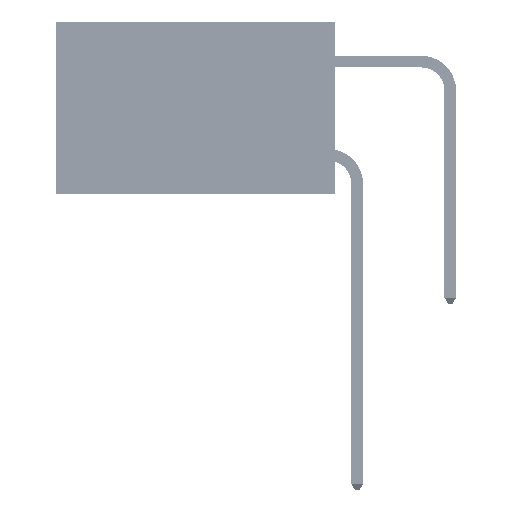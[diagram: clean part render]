
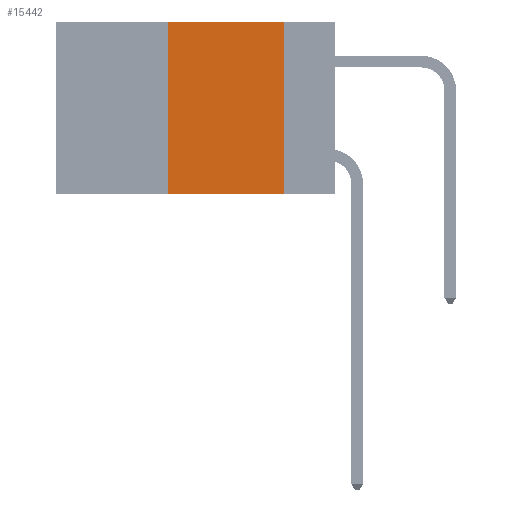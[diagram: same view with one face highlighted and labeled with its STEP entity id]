
A CAD part, left-side view. The second image highlights one B-rep face of the part: STEP entity #15442.
In plain terms, the highlighted planar face has unit normal (-1, 0, 0).
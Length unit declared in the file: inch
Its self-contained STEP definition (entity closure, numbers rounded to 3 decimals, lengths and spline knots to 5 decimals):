
#2780 = DIRECTION ( 'NONE',  ( 0., 0., 1. ) ) ;
#3039 = CARTESIAN_POINT ( 'NONE',  ( 0., 0.6, -0.37 ) ) ;
#4816 = CARTESIAN_POINT ( 'NONE',  ( 0., 0.36, -0.37 ) ) ;
#5075 = CARTESIAN_POINT ( 'NONE',  ( 0., 0.6, 0. ) ) ;
#6278 = VECTOR ( 'NONE', #37087, 39.37008 ) ;
#7468 = CARTESIAN_POINT ( 'NONE',  ( 0., 0.36, 0. ) ) ;
#8004 = CARTESIAN_POINT ( 'NONE',  ( 0., 0.11, -0.37 ) ) ;
#8449 = EDGE_LOOP ( 'NONE', ( #29935, #36729, #36062, #20959 ) ) ;
#8723 = DIRECTION ( 'NONE',  ( 1., 0., 0. ) ) ;
#8967 = FACE_OUTER_BOUND ( 'NONE', #8449, .T. ) ;
#9272 = VECTOR ( 'NONE', #2780, 39.37008 ) ;
#11995 = EDGE_CURVE ( 'NONE', #47889, #17539, #29775, .T. ) ;
#12597 = AXIS2_PLACEMENT_3D ( 'NONE', #16553, #8723, #31439 ) ;
#14739 = VECTOR ( 'NONE', #44502, 39.37008 ) ;
#15414 = EDGE_CURVE ( 'NONE', #46195, #47889, #27761, .T. ) ;
#15442 = ADVANCED_FACE ( 'NONE', ( #8967 ), #35083, .F. ) ;
#16553 = CARTESIAN_POINT ( 'NONE',  ( 0., 0.6, 0. ) ) ;
#17539 = VERTEX_POINT ( 'NONE', #8004 ) ;
#20959 = ORIENTED_EDGE ( 'NONE', *, *, #37553, .T. ) ;
#21568 = LINE ( 'NONE', #36219, #9272 ) ;
#25056 = VECTOR ( 'NONE', #39238, 39.37008 ) ;
#26111 = CARTESIAN_POINT ( 'NONE',  ( 0., 0.11, 0. ) ) ;
#27717 = VERTEX_POINT ( 'NONE', #4816 ) ;
#27761 = LINE ( 'NONE', #5075, #25056 ) ;
#29775 = LINE ( 'NONE', #26111, #6278 ) ;
#29935 = ORIENTED_EDGE ( 'NONE', *, *, #11995, .F. ) ;
#31439 = DIRECTION ( 'NONE',  ( 0., 0., -1. ) ) ;
#32326 = CARTESIAN_POINT ( 'NONE',  ( 0., 0.11, 0. ) ) ;
#35083 = PLANE ( 'NONE',  #12597 ) ;
#36062 = ORIENTED_EDGE ( 'NONE', *, *, #38162, .F. ) ;
#36219 = CARTESIAN_POINT ( 'NONE',  ( 0., 0.36, 0. ) ) ;
#36729 = ORIENTED_EDGE ( 'NONE', *, *, #15414, .F. ) ;
#37087 = DIRECTION ( 'NONE',  ( 0., 0., -1. ) ) ;
#37553 = EDGE_CURVE ( 'NONE', #27717, #17539, #47921, .T. ) ;
#38162 = EDGE_CURVE ( 'NONE', #27717, #46195, #21568, .T. ) ;
#39238 = DIRECTION ( 'NONE',  ( 0., -1., 0. ) ) ;
#44502 = DIRECTION ( 'NONE',  ( 0., -1., 0. ) ) ;
#46195 = VERTEX_POINT ( 'NONE', #7468 ) ;
#47889 = VERTEX_POINT ( 'NONE', #32326 ) ;
#47921 = LINE ( 'NONE', #3039, #14739 ) ;
